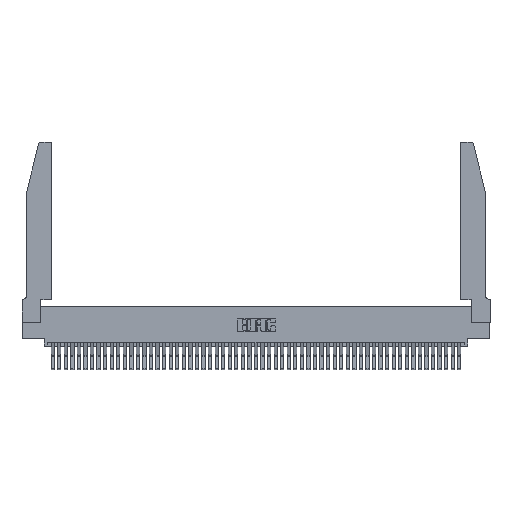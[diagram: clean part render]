
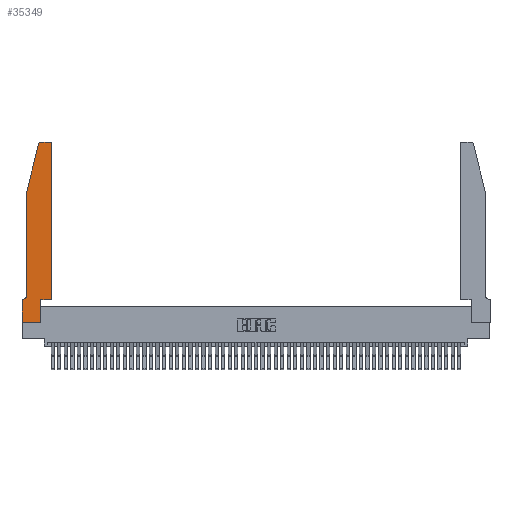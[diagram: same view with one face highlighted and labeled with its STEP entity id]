
A CAD part, top view. The second image highlights one B-rep face of the part: STEP entity #35349.
In plain terms, the highlighted planar face has unit normal (0, 0, 1).
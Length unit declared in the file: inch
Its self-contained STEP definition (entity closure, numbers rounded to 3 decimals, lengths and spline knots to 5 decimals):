
#137 = CARTESIAN_POINT ( 'NONE',  ( 0.2865, 0.35, 0.37 ) ) ;
#413 = LINE ( 'NONE', #137, #41581 ) ;
#696 = EDGE_CURVE ( 'NONE', #21245, #46072, #44821, .T. ) ;
#999 = EDGE_CURVE ( 'NONE', #28909, #36757, #30051, .T. ) ;
#1134 = CARTESIAN_POINT ( 'NONE',  ( 0.0755, 0.35, 0.37 ) ) ;
#1327 = CIRCLE ( 'NONE', #19427, 0.03 ) ;
#1381 = ORIENTED_EDGE ( 'NONE', *, *, #46052, .T. ) ;
#1451 = CARTESIAN_POINT ( 'NONE',  ( 0.0755, 2., 0.37 ) ) ;
#1552 = ORIENTED_EDGE ( 'NONE', *, *, #51102, .T. ) ;
#1778 = DIRECTION ( 'NONE',  ( -0.239, -0.971, 0. ) ) ;
#1998 = CARTESIAN_POINT ( 'NONE',  ( 0.4505, 0.35, 0.37 ) ) ;
#2398 = VERTEX_POINT ( 'NONE', #12219 ) ;
#3409 = CARTESIAN_POINT ( 'NONE',  ( 0.0755, 0.42, 0.37 ) ) ;
#4206 = VECTOR ( 'NONE', #25652, 39.37008 ) ;
#4578 = LINE ( 'NONE', #1134, #15387 ) ;
#5479 = LINE ( 'NONE', #29598, #4206 ) ;
#6884 = CARTESIAN_POINT ( 'NONE',  ( 0.4205, 2.75, 0.37 ) ) ;
#7562 = EDGE_CURVE ( 'NONE', #34416, #28909, #4578, .T. ) ;
#7784 = VERTEX_POINT ( 'NONE', #39121 ) ;
#8284 = ORIENTED_EDGE ( 'NONE', *, *, #696, .T. ) ;
#8677 = ORIENTED_EDGE ( 'NONE', *, *, #999, .T. ) ;
#8843 = DIRECTION ( 'NONE',  ( 1., 0., 0. ) ) ;
#8957 = ORIENTED_EDGE ( 'NONE', *, *, #32325, .T. ) ;
#9802 = VECTOR ( 'NONE', #1778, 39.37008 ) ;
#10389 = PLANE ( 'NONE',  #23436 ) ;
#10681 = EDGE_CURVE ( 'NONE', #46072, #40395, #20071, .T. ) ;
#12219 = CARTESIAN_POINT ( 'NONE',  ( 0.2865, 0.35, 0.37 ) ) ;
#13388 = CARTESIAN_POINT ( 'NONE',  ( 0.4505, 2.72, 0.37 ) ) ;
#13448 = DIRECTION ( 'NONE',  ( 0., -1., 0. ) ) ;
#13902 = FACE_OUTER_BOUND ( 'NONE', #51485, .T. ) ;
#14478 = DIRECTION ( 'NONE',  ( 0., 0., 1. ) ) ;
#15387 = VECTOR ( 'NONE', #25275, 39.37008 ) ;
#16214 = DIRECTION ( 'NONE',  ( 0., 0., -1. ) ) ;
#17054 = ORIENTED_EDGE ( 'NONE', *, *, #7562, .T. ) ;
#17254 = LINE ( 'NONE', #1998, #36950 ) ;
#17520 = LINE ( 'NONE', #32695, #28018 ) ;
#18767 = AXIS2_PLACEMENT_3D ( 'NONE', #42636, #19107, #46577 ) ;
#19107 = DIRECTION ( 'NONE',  ( 0., 0., 1. ) ) ;
#19229 = CARTESIAN_POINT ( 'NONE',  ( 0.0755, 2., 0.37 ) ) ;
#19427 = AXIS2_PLACEMENT_3D ( 'NONE', #46412, #22901, #50449 ) ;
#19501 = AXIS2_PLACEMENT_3D ( 'NONE', #39809, #16214, #43754 ) ;
#20071 = LINE ( 'NONE', #27008, #39732 ) ;
#21245 = VERTEX_POINT ( 'NONE', #13388 ) ;
#21784 = DIRECTION ( 'NONE',  ( 0., -1., 0. ) ) ;
#22744 = CARTESIAN_POINT ( 'NONE',  ( 0.284, 2.75, 0.37 ) ) ;
#22901 = DIRECTION ( 'NONE',  ( 0., 0., 1. ) ) ;
#23056 = VERTEX_POINT ( 'NONE', #30579 ) ;
#23436 = AXIS2_PLACEMENT_3D ( 'NONE', #49850, #14478, #42060 ) ;
#24675 = DIRECTION ( 'NONE',  ( 0., 1., 0. ) ) ;
#25006 = EDGE_CURVE ( 'NONE', #35571, #34416, #41362, .T. ) ;
#25275 = DIRECTION ( 'NONE',  ( -1., 0., 0. ) ) ;
#25469 = EDGE_CURVE ( 'NONE', #46789, #35571, #50605, .T. ) ;
#25652 = DIRECTION ( 'NONE',  ( 0., 1., 0. ) ) ;
#27008 = CARTESIAN_POINT ( 'NONE',  ( 0.2605, 2.75, 0.37 ) ) ;
#27283 = ORIENTED_EDGE ( 'NONE', *, *, #25006, .T. ) ;
#27774 = CARTESIAN_POINT ( 'NONE',  ( 0.4505, 0.35, 0.37 ) ) ;
#28018 = VECTOR ( 'NONE', #8843, 39.37008 ) ;
#28099 = CARTESIAN_POINT ( 'NONE',  ( 0.0055, 0.35, 0.37 ) ) ;
#28909 = VERTEX_POINT ( 'NONE', #43904 ) ;
#29079 = CARTESIAN_POINT ( 'NONE',  ( 0., 0., 0.37 ) ) ;
#29498 = ORIENTED_EDGE ( 'NONE', *, *, #10681, .T. ) ;
#29598 = CARTESIAN_POINT ( 'NONE',  ( 0.4505, 0.35, 0.37 ) ) ;
#30051 = LINE ( 'NONE', #29079, #49719 ) ;
#30063 = DIRECTION ( 'NONE',  ( 1., 0., 0. ) ) ;
#30579 = CARTESIAN_POINT ( 'NONE',  ( 0.25487, 2.72718, 0.37 ) ) ;
#32325 = EDGE_CURVE ( 'NONE', #47603, #21245, #5479, .T. ) ;
#32695 = CARTESIAN_POINT ( 'NONE',  ( 0., 0., 0.37 ) ) ;
#32996 = EDGE_CURVE ( 'NONE', #2398, #47603, #17254, .T. ) ;
#34416 = VERTEX_POINT ( 'NONE', #28099 ) ;
#34986 = ORIENTED_EDGE ( 'NONE', *, *, #25469, .T. ) ;
#35349 = ADVANCED_FACE ( 'NONE', ( #13902 ), #10389, .T. ) ;
#35571 = VERTEX_POINT ( 'NONE', #3409 ) ;
#36289 = EDGE_CURVE ( 'NONE', #7784, #2398, #413, .T. ) ;
#36757 = VERTEX_POINT ( 'NONE', #39003 ) ;
#36950 = VECTOR ( 'NONE', #30063, 39.37008 ) ;
#36995 = ORIENTED_EDGE ( 'NONE', *, *, #36289, .T. ) ;
#37029 = EDGE_CURVE ( 'NONE', #36757, #7784, #17520, .T. ) ;
#38790 = DIRECTION ( 'NONE',  ( -1., 0., 0. ) ) ;
#39003 = CARTESIAN_POINT ( 'NONE',  ( 0., 0., 0.37 ) ) ;
#39121 = CARTESIAN_POINT ( 'NONE',  ( 0.2865, 0., 0.37 ) ) ;
#39732 = VECTOR ( 'NONE', #38790, 39.37008 ) ;
#39809 = CARTESIAN_POINT ( 'NONE',  ( 0.0055, 0.42, 0.37 ) ) ;
#40088 = VECTOR ( 'NONE', #21784, 39.37008 ) ;
#40395 = VERTEX_POINT ( 'NONE', #22744 ) ;
#41362 = CIRCLE ( 'NONE', #19501, 0.07 ) ;
#41398 = LINE ( 'NONE', #49440, #9802 ) ;
#41581 = VECTOR ( 'NONE', #24675, 39.37008 ) ;
#42060 = DIRECTION ( 'NONE',  ( 1., 0., 0. ) ) ;
#42636 = CARTESIAN_POINT ( 'NONE',  ( 0.4205, 2.72, 0.37 ) ) ;
#43754 = DIRECTION ( 'NONE',  ( -1., 0., 0. ) ) ;
#43904 = CARTESIAN_POINT ( 'NONE',  ( 0., 0.35, 0.37 ) ) ;
#44295 = ORIENTED_EDGE ( 'NONE', *, *, #32996, .T. ) ;
#44821 = CIRCLE ( 'NONE', #18767, 0.03 ) ;
#46052 = EDGE_CURVE ( 'NONE', #40395, #23056, #1327, .T. ) ;
#46072 = VERTEX_POINT ( 'NONE', #6884 ) ;
#46412 = CARTESIAN_POINT ( 'NONE',  ( 0.284, 2.72, 0.37 ) ) ;
#46577 = DIRECTION ( 'NONE',  ( 1., 0., 0. ) ) ;
#46789 = VERTEX_POINT ( 'NONE', #19229 ) ;
#47603 = VERTEX_POINT ( 'NONE', #27774 ) ;
#48832 = ORIENTED_EDGE ( 'NONE', *, *, #37029, .T. ) ;
#49440 = CARTESIAN_POINT ( 'NONE',  ( 0.0755, 2., 0.37 ) ) ;
#49719 = VECTOR ( 'NONE', #13448, 39.37008 ) ;
#49850 = CARTESIAN_POINT ( 'NONE',  ( 0., 0.35, 0.37 ) ) ;
#50449 = DIRECTION ( 'NONE',  ( 1., 0., 0. ) ) ;
#50605 = LINE ( 'NONE', #1451, #40088 ) ;
#51102 = EDGE_CURVE ( 'NONE', #23056, #46789, #41398, .T. ) ;
#51485 = EDGE_LOOP ( 'NONE', ( #29498, #1381, #1552, #34986, #27283, #17054, #8677, #48832, #36995, #44295, #8957, #8284 ) ) ;
